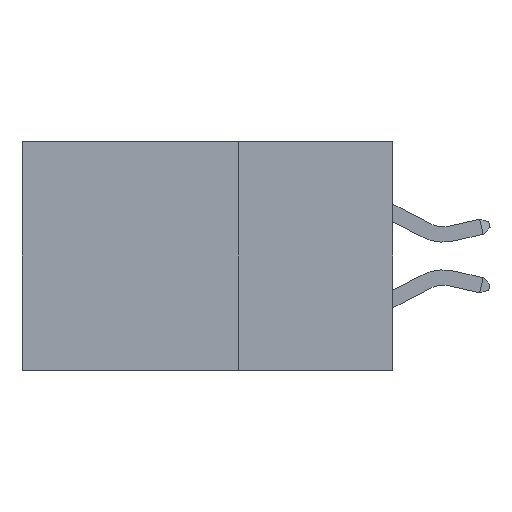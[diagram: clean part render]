
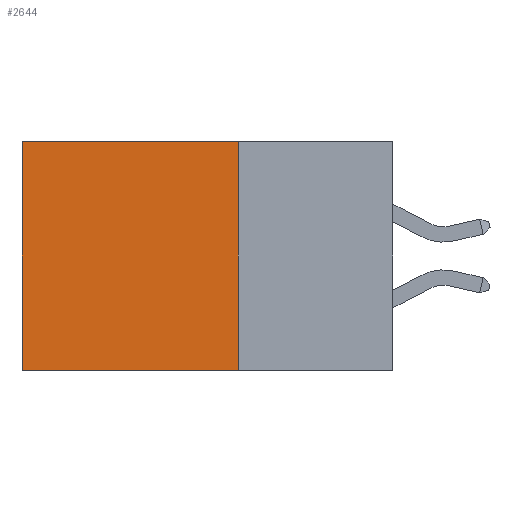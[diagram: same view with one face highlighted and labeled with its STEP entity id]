
A CAD part, left-side view. The second image highlights one B-rep face of the part: STEP entity #2644.
In plain terms, the highlighted planar face has unit normal (-1, 0, 0).
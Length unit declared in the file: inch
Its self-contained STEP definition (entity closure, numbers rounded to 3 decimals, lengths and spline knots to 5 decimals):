
#33 = LINE ( 'NONE', #6370, #533 ) ;
#360 = VERTEX_POINT ( 'NONE', #7109 ) ;
#533 = VECTOR ( 'NONE', #6566, 39.37008 ) ;
#600 = DIRECTION ( 'NONE',  ( 0., 1., 0. ) ) ;
#964 = CARTESIAN_POINT ( 'NONE',  ( 0.2875, 0.25, 0. ) ) ;
#1286 = EDGE_CURVE ( 'NONE', #4166, #8751, #3517, .T. ) ;
#1353 = DIRECTION ( 'NONE',  ( 0., 0., -1. ) ) ;
#1372 = CARTESIAN_POINT ( 'NONE',  ( 0.2875, 0.6, 0. ) ) ;
#2017 = FACE_OUTER_BOUND ( 'NONE', #2889, .T. ) ;
#2644 = ADVANCED_FACE ( 'NONE', ( #2017 ), #7311, .F. ) ;
#2889 = EDGE_LOOP ( 'NONE', ( #4106, #7978, #2909, #6852 ) ) ;
#2909 = ORIENTED_EDGE ( 'NONE', *, *, #5805, .F. ) ;
#3304 = VECTOR ( 'NONE', #4210, 39.37008 ) ;
#3517 = LINE ( 'NONE', #4755, #3304 ) ;
#3685 = LINE ( 'NONE', #964, #7381 ) ;
#3789 = DIRECTION ( 'NONE',  ( 0., 0., -1. ) ) ;
#4106 = ORIENTED_EDGE ( 'NONE', *, *, #6858, .T. ) ;
#4166 = VERTEX_POINT ( 'NONE', #5815 ) ;
#4210 = DIRECTION ( 'NONE',  ( 0., 1., 0. ) ) ;
#4755 = CARTESIAN_POINT ( 'NONE',  ( 0.2875, 0.25, -0.37 ) ) ;
#5204 = EDGE_CURVE ( 'NONE', #360, #7592, #3685, .T. ) ;
#5344 = CARTESIAN_POINT ( 'NONE',  ( 0.2875, 0.25, 0. ) ) ;
#5419 = AXIS2_PLACEMENT_3D ( 'NONE', #5344, #7297, #3789 ) ;
#5725 = LINE ( 'NONE', #1372, #9074 ) ;
#5805 = EDGE_CURVE ( 'NONE', #360, #4166, #33, .T. ) ;
#5815 = CARTESIAN_POINT ( 'NONE',  ( 0.2875, 0.25, -0.37 ) ) ;
#6370 = CARTESIAN_POINT ( 'NONE',  ( 0.2875, 0.25, 0. ) ) ;
#6458 = CARTESIAN_POINT ( 'NONE',  ( 0.2875, 0.6, 0. ) ) ;
#6566 = DIRECTION ( 'NONE',  ( 0., 0., -1. ) ) ;
#6852 = ORIENTED_EDGE ( 'NONE', *, *, #5204, .T. ) ;
#6858 = EDGE_CURVE ( 'NONE', #7592, #8751, #5725, .T. ) ;
#7109 = CARTESIAN_POINT ( 'NONE',  ( 0.2875, 0.25, 0. ) ) ;
#7297 = DIRECTION ( 'NONE',  ( 1., 0., 0. ) ) ;
#7311 = PLANE ( 'NONE',  #5419 ) ;
#7381 = VECTOR ( 'NONE', #600, 39.37008 ) ;
#7592 = VERTEX_POINT ( 'NONE', #6458 ) ;
#7835 = CARTESIAN_POINT ( 'NONE',  ( 0.2875, 0.6, -0.37 ) ) ;
#7978 = ORIENTED_EDGE ( 'NONE', *, *, #1286, .F. ) ;
#8751 = VERTEX_POINT ( 'NONE', #7835 ) ;
#9074 = VECTOR ( 'NONE', #1353, 39.37008 ) ;
